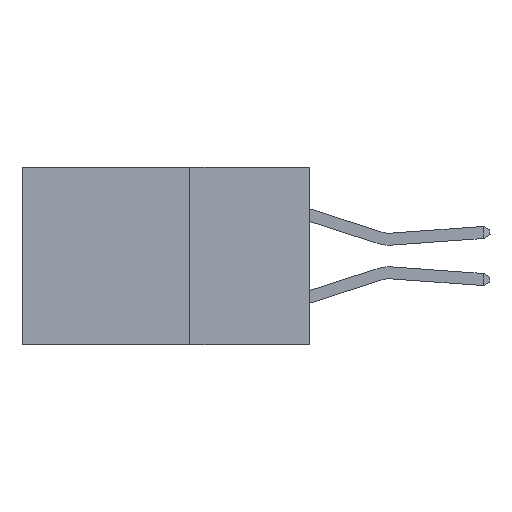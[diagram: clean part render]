
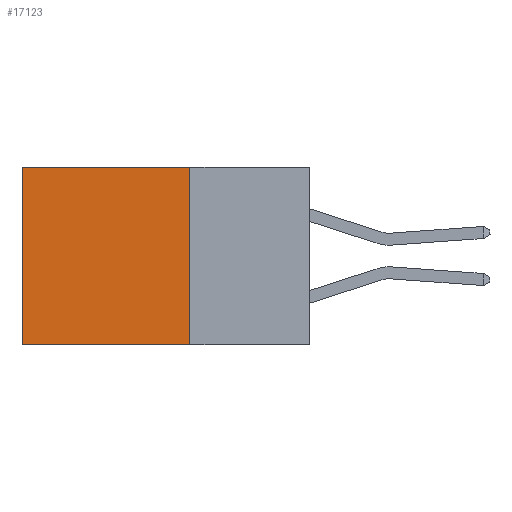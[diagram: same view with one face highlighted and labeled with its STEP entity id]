
A CAD part, left-side view. The second image highlights one B-rep face of the part: STEP entity #17123.
In plain terms, the highlighted planar face has unit normal (-1, 0, 0).
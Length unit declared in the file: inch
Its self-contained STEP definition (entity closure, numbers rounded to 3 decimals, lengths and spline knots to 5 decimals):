
#1058 = ORIENTED_EDGE ( 'NONE', *, *, #10980, .F. ) ;
#1297 = LINE ( 'NONE', #32740, #29619 ) ;
#2685 = LINE ( 'NONE', #25112, #22741 ) ;
#3554 = VERTEX_POINT ( 'NONE', #12555 ) ;
#4279 = VERTEX_POINT ( 'NONE', #14164 ) ;
#4995 = ORIENTED_EDGE ( 'NONE', *, *, #29171, .F. ) ;
#5163 = VECTOR ( 'NONE', #11026, 39.37008 ) ;
#5373 = DIRECTION ( 'NONE',  ( 0., 0., -1. ) ) ;
#5997 = LINE ( 'NONE', #19518, #5163 ) ;
#6363 = DIRECTION ( 'NONE',  ( 0., 0., -1. ) ) ;
#8754 = FACE_OUTER_BOUND ( 'NONE', #23499, .T. ) ;
#9596 = CARTESIAN_POINT ( 'NONE',  ( 0.298, 0.6, 0. ) ) ;
#10256 = ORIENTED_EDGE ( 'NONE', *, *, #10882, .T. ) ;
#10882 = EDGE_CURVE ( 'NONE', #18534, #4279, #5997, .T. ) ;
#10980 = EDGE_CURVE ( 'NONE', #12121, #4279, #2685, .T. ) ;
#11026 = DIRECTION ( 'NONE',  ( 0., 0., -1. ) ) ;
#11141 = CARTESIAN_POINT ( 'NONE',  ( 0.298, 0.25, 0. ) ) ;
#11973 = VECTOR ( 'NONE', #27199, 39.37008 ) ;
#12121 = VERTEX_POINT ( 'NONE', #16855 ) ;
#12555 = CARTESIAN_POINT ( 'NONE',  ( 0.298, 0.25, 0. ) ) ;
#14116 = ORIENTED_EDGE ( 'NONE', *, *, #30192, .T. ) ;
#14164 = CARTESIAN_POINT ( 'NONE',  ( 0.298, 0.6, -0.37 ) ) ;
#14507 = DIRECTION ( 'NONE',  ( 0., 1., 0. ) ) ;
#16855 = CARTESIAN_POINT ( 'NONE',  ( 0.298, 0.25, -0.37 ) ) ;
#16915 = CARTESIAN_POINT ( 'NONE',  ( 0.298, 0.25, 0. ) ) ;
#17123 = ADVANCED_FACE ( 'NONE', ( #8754 ), #27098, .F. ) ;
#18534 = VERTEX_POINT ( 'NONE', #9596 ) ;
#19518 = CARTESIAN_POINT ( 'NONE',  ( 0.298, 0.6, 0. ) ) ;
#22686 = AXIS2_PLACEMENT_3D ( 'NONE', #11141, #29751, #5373 ) ;
#22741 = VECTOR ( 'NONE', #14507, 39.37008 ) ;
#23499 = EDGE_LOOP ( 'NONE', ( #10256, #1058, #4995, #14116 ) ) ;
#25112 = CARTESIAN_POINT ( 'NONE',  ( 0.298, 0.25, -0.37 ) ) ;
#27098 = PLANE ( 'NONE',  #22686 ) ;
#27199 = DIRECTION ( 'NONE',  ( 0., 1., 0. ) ) ;
#29171 = EDGE_CURVE ( 'NONE', #3554, #12121, #1297, .T. ) ;
#29619 = VECTOR ( 'NONE', #6363, 39.37008 ) ;
#29751 = DIRECTION ( 'NONE',  ( 1., 0., 0. ) ) ;
#30192 = EDGE_CURVE ( 'NONE', #3554, #18534, #34442, .T. ) ;
#32740 = CARTESIAN_POINT ( 'NONE',  ( 0.298, 0.25, 0. ) ) ;
#34442 = LINE ( 'NONE', #16915, #11973 ) ;
